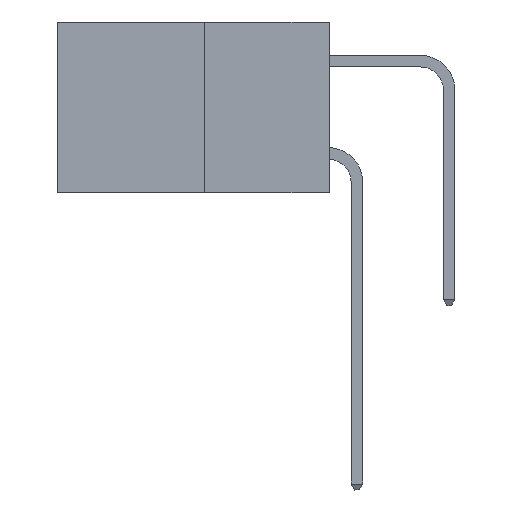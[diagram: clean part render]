
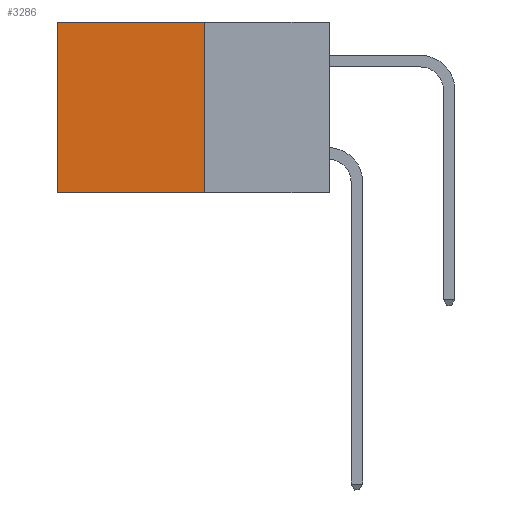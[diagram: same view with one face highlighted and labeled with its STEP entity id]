
A CAD part, left-side view. The second image highlights one B-rep face of the part: STEP entity #3286.
In plain terms, the highlighted planar face has unit normal (-1, 0, 0).
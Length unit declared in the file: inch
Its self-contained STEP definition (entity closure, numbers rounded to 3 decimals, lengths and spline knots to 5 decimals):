
#120 = ORIENTED_EDGE ( 'NONE', *, *, #10160, .F. ) ;
#429 = DIRECTION ( 'NONE',  ( 0., 1., 0. ) ) ;
#747 = ORIENTED_EDGE ( 'NONE', *, *, #7862, .T. ) ;
#851 = DIRECTION ( 'NONE',  ( 0., 0., -1. ) ) ;
#1083 = DIRECTION ( 'NONE',  ( 0., 1., 0. ) ) ;
#1132 = CARTESIAN_POINT ( 'NONE',  ( 0.277, 0.27, 0. ) ) ;
#1291 = CARTESIAN_POINT ( 'NONE',  ( 0.277, 0.59, 0. ) ) ;
#2577 = ORIENTED_EDGE ( 'NONE', *, *, #8823, .F. ) ;
#2700 = VERTEX_POINT ( 'NONE', #6097 ) ;
#2826 = CARTESIAN_POINT ( 'NONE',  ( 0.277, 0.59, -0.37 ) ) ;
#2908 = LINE ( 'NONE', #2826, #5225 ) ;
#3254 = ORIENTED_EDGE ( 'NONE', *, *, #9778, .T. ) ;
#3286 = ADVANCED_FACE ( 'NONE', ( #4049 ), #5790, .F. ) ;
#3420 = CARTESIAN_POINT ( 'NONE',  ( 0.277, 0.27, -0.37 ) ) ;
#3429 = DIRECTION ( 'NONE',  ( 0., 0., -1. ) ) ;
#3488 = LINE ( 'NONE', #1132, #6059 ) ;
#4049 = FACE_OUTER_BOUND ( 'NONE', #10307, .T. ) ;
#5015 = VERTEX_POINT ( 'NONE', #1291 ) ;
#5178 = VERTEX_POINT ( 'NONE', #11882 ) ;
#5225 = VECTOR ( 'NONE', #851, 39.37008 ) ;
#5739 = VECTOR ( 'NONE', #429, 39.37008 ) ;
#5790 = PLANE ( 'NONE',  #10653 ) ;
#5809 = VERTEX_POINT ( 'NONE', #6357 ) ;
#6059 = VECTOR ( 'NONE', #1083, 39.37008 ) ;
#6097 = CARTESIAN_POINT ( 'NONE',  ( 0.277, 0.59, -0.37 ) ) ;
#6357 = CARTESIAN_POINT ( 'NONE',  ( 0.277, 0.27, 0. ) ) ;
#6698 = DIRECTION ( 'NONE',  ( 0., 0., -1. ) ) ;
#7769 = VECTOR ( 'NONE', #3429, 39.37008 ) ;
#7862 = EDGE_CURVE ( 'NONE', #5809, #5015, #3488, .T. ) ;
#7868 = DIRECTION ( 'NONE',  ( 1., 0., 0. ) ) ;
#8342 = LINE ( 'NONE', #3420, #5739 ) ;
#8823 = EDGE_CURVE ( 'NONE', #5178, #2700, #8342, .T. ) ;
#9778 = EDGE_CURVE ( 'NONE', #5015, #2700, #2908, .T. ) ;
#10160 = EDGE_CURVE ( 'NONE', #5809, #5178, #10456, .T. ) ;
#10307 = EDGE_LOOP ( 'NONE', ( #3254, #2577, #120, #747 ) ) ;
#10456 = LINE ( 'NONE', #12206, #7769 ) ;
#10653 = AXIS2_PLACEMENT_3D ( 'NONE', #11320, #7868, #6698 ) ;
#11320 = CARTESIAN_POINT ( 'NONE',  ( 0.277, 0.27, -0.37 ) ) ;
#11882 = CARTESIAN_POINT ( 'NONE',  ( 0.277, 0.27, -0.37 ) ) ;
#12206 = CARTESIAN_POINT ( 'NONE',  ( 0.277, 0.27, -0.37 ) ) ;
